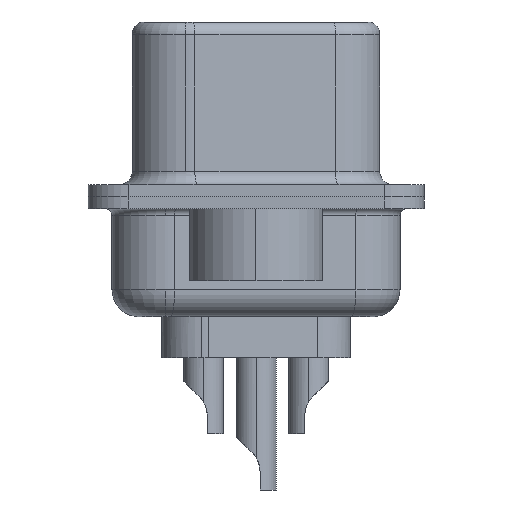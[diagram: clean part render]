
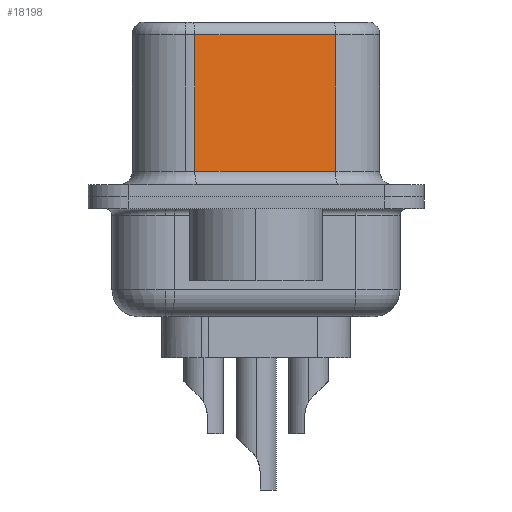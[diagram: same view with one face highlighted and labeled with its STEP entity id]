
A CAD part, left-side view. The second image highlights one B-rep face of the part: STEP entity #18198.
In plain terms, the highlighted planar face has unit normal (-0.985, -0.174, 0).
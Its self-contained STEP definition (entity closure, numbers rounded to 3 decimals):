
#384 = AXIS2_PLACEMENT_3D ( 'NONE', #20357, #20137, #16752 ) ;
#468 = ORIENTED_EDGE ( 'NONE', *, *, #22079, .F. ) ;
#919 = DIRECTION ( 'NONE',  ( 0., 0., -1. ) ) ;
#1727 = VECTOR ( 'NONE', #8301, 1000. ) ;
#3035 = EDGE_CURVE ( 'NONE', #18535, #5558, #12153, .T. ) ;
#3088 = CARTESIAN_POINT ( 'NONE',  ( 3.615, 2.293, 6.57 ) ) ;
#3102 = CARTESIAN_POINT ( 'NONE',  ( 4.546, -2.987, 6.07 ) ) ;
#3388 = EDGE_CURVE ( 'NONE', #10498, #18535, #15434, .T. ) ;
#3844 = ORIENTED_EDGE ( 'NONE', *, *, #5839, .T. ) ;
#4082 = EDGE_LOOP ( 'NONE', ( #468, #3844, #13397, #16872 ) ) ;
#4092 = CARTESIAN_POINT ( 'NONE',  ( 3.615, 2.293, 0.95 ) ) ;
#4820 = CARTESIAN_POINT ( 'NONE',  ( 4.546, -2.987, 0.95 ) ) ;
#4822 = LINE ( 'NONE', #6858, #1727 ) ;
#5558 = VERTEX_POINT ( 'NONE', #11215 ) ;
#5839 = EDGE_CURVE ( 'NONE', #23084, #10498, #4822, .T. ) ;
#6065 = CARTESIAN_POINT ( 'NONE',  ( 4.546, -2.987, 6.57 ) ) ;
#6858 = CARTESIAN_POINT ( 'NONE',  ( 4.546, -2.987, 6.07 ) ) ;
#6866 = CARTESIAN_POINT ( 'NONE',  ( 3.615, 2.293, 6.07 ) ) ;
#8301 = DIRECTION ( 'NONE',  ( -0.174, 0.985, 0. ) ) ;
#9219 = FACE_OUTER_BOUND ( 'NONE', #4082, .T. ) ;
#10498 = VERTEX_POINT ( 'NONE', #6866 ) ;
#11215 = CARTESIAN_POINT ( 'NONE',  ( 4.546, -2.987, 0.95 ) ) ;
#12153 = LINE ( 'NONE', #4820, #13543 ) ;
#13397 = ORIENTED_EDGE ( 'NONE', *, *, #3388, .T. ) ;
#13543 = VECTOR ( 'NONE', #14309, 1000. ) ;
#14309 = DIRECTION ( 'NONE',  ( 0.174, -0.985, 0. ) ) ;
#15434 = LINE ( 'NONE', #3088, #20081 ) ;
#15535 = LINE ( 'NONE', #6065, #16740 ) ;
#16740 = VECTOR ( 'NONE', #16857, 1000. ) ;
#16752 = DIRECTION ( 'NONE',  ( -0.174, 0.985, 0. ) ) ;
#16857 = DIRECTION ( 'NONE',  ( 0., 0., -1. ) ) ;
#16868 = PLANE ( 'NONE',  #384 ) ;
#16872 = ORIENTED_EDGE ( 'NONE', *, *, #3035, .T. ) ;
#18198 = ADVANCED_FACE ( 'NONE', ( #9219 ), #16868, .F. ) ;
#18535 = VERTEX_POINT ( 'NONE', #4092 ) ;
#20081 = VECTOR ( 'NONE', #919, 1000. ) ;
#20137 = DIRECTION ( 'NONE',  ( 0.985, 0.174, 0. ) ) ;
#20357 = CARTESIAN_POINT ( 'NONE',  ( 4.546, -2.987, 6.57 ) ) ;
#22079 = EDGE_CURVE ( 'NONE', #23084, #5558, #15535, .T. ) ;
#23084 = VERTEX_POINT ( 'NONE', #3102 ) ;
